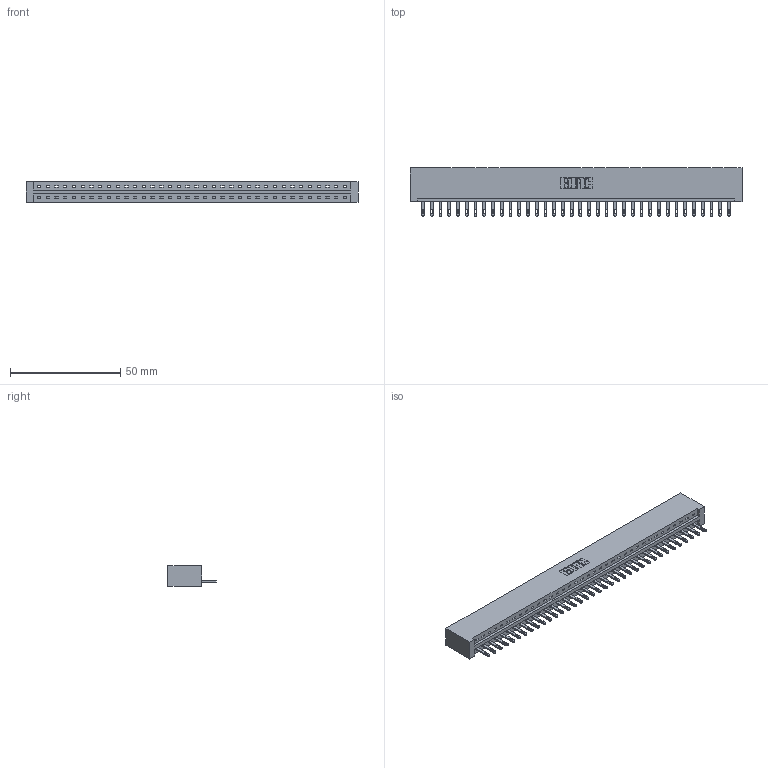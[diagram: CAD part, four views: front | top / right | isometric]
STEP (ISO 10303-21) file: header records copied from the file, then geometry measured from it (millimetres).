
FILE_DESCRIPTION (( 'STEP AP203' ), '1' );
FILE_NAME ('337-036-500-101.STEP', '2019-10-01T13:31:16', ( '' ), ( '' ), 'SwSTEP 2.0', 'SolidWorks 2016', '' );
FILE_SCHEMA (( 'CONFIG_CONTROL_DESIGN' ));
Length unit declared in the file: inch
Products named in the file (3): 345-292-001_345-293-100; 337 Part_No Mounting Lugs; 337-036-500-101
Assembly tree (37 placements, depth 2):
  337-036-500-101
    337 Part_No Mounting Lugs
    345-292-001_345-293-100  x36
Bounding box: 150.52 x 21.85 x 9.4 mm (x, y, z)
Volume: 16330 mm3; surface area: 16906.8 mm2
Topology: 37 solids, 37 shells, 2194 faces, 6767 edges, 4510 vertices
Faces by surface type: plane 1506, cylinder 688
Entity records: 27189 total; most frequent: CARTESIAN_POINT 4742, ORIENTED_EDGE 4714, DIRECTION 3997, EDGE_CURVE 2357, LINE 2233, VECTOR 2233, VERTEX_POINT 1570, AXIS2_PLACEMENT_3D 882
